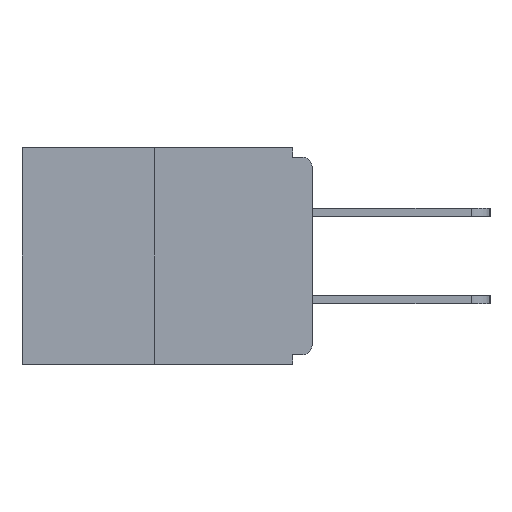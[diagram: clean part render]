
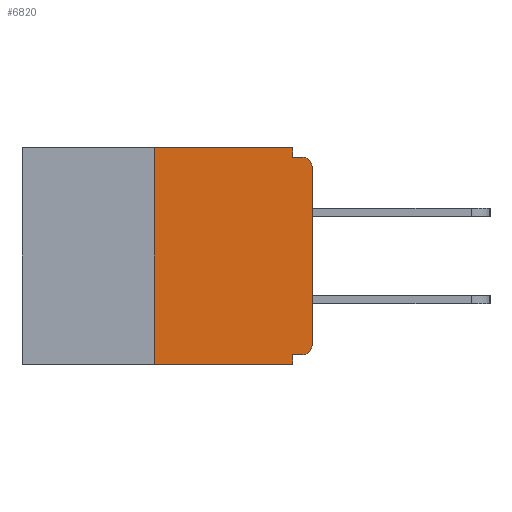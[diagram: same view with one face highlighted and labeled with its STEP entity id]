
A CAD part, left-side view. The second image highlights one B-rep face of the part: STEP entity #6820.
In plain terms, the highlighted planar face has unit normal (-1, 0, 0).
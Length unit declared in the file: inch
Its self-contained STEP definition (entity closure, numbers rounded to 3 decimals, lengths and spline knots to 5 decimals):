
#586 = VERTEX_POINT ( 'NONE', #4820 ) ;
#760 = CARTESIAN_POINT ( 'NONE',  ( 0., 0.015, -0.313 ) ) ;
#1252 = LINE ( 'NONE', #9778, #4649 ) ;
#1387 = VECTOR ( 'NONE', #11761, 39.37008 ) ;
#1599 = EDGE_CURVE ( 'NONE', #7360, #13210, #11874, .T. ) ;
#1698 = CARTESIAN_POINT ( 'NONE',  ( 0., 0.46, 0. ) ) ;
#1788 = EDGE_CURVE ( 'NONE', #4727, #586, #2448, .T. ) ;
#2043 = ORIENTED_EDGE ( 'NONE', *, *, #12614, .F. ) ;
#2048 = LINE ( 'NONE', #6075, #18670 ) ;
#2087 = VERTEX_POINT ( 'NONE', #13366 ) ;
#2448 = CIRCLE ( 'NONE', #17459, 0.015 ) ;
#2493 = DIRECTION ( 'NONE',  ( 0., 0., -1. ) ) ;
#2789 = DIRECTION ( 'NONE',  ( 0., -1., 0. ) ) ;
#2882 = DIRECTION ( 'NONE',  ( 0., 1., 0. ) ) ;
#3087 = VERTEX_POINT ( 'NONE', #14755 ) ;
#3408 = VERTEX_POINT ( 'NONE', #15895 ) ;
#3495 = LINE ( 'NONE', #4581, #8806 ) ;
#3751 = DIRECTION ( 'NONE',  ( -1., 0., 0. ) ) ;
#3957 = CIRCLE ( 'NONE', #9616, 0.015 ) ;
#4191 = CARTESIAN_POINT ( 'NONE',  ( 0., 0., -0.015 ) ) ;
#4308 = FACE_OUTER_BOUND ( 'NONE', #7816, .T. ) ;
#4376 = EDGE_CURVE ( 'NONE', #586, #6643, #3495, .T. ) ;
#4581 = CARTESIAN_POINT ( 'NONE',  ( 0., 0., 0. ) ) ;
#4649 = VECTOR ( 'NONE', #2882, 39.37008 ) ;
#4727 = VERTEX_POINT ( 'NONE', #10155 ) ;
#4807 = VECTOR ( 'NONE', #6513, 39.37008 ) ;
#4820 = CARTESIAN_POINT ( 'NONE',  ( 0., 0., -0.313 ) ) ;
#4939 = EDGE_CURVE ( 'NONE', #2087, #3087, #7409, .T. ) ;
#5169 = AXIS2_PLACEMENT_3D ( 'NONE', #1698, #14975, #18326 ) ;
#5762 = EDGE_CURVE ( 'NONE', #16862, #3087, #15166, .T. ) ;
#6075 = CARTESIAN_POINT ( 'NONE',  ( 0., 0.25, 0. ) ) ;
#6101 = ORIENTED_EDGE ( 'NONE', *, *, #18833, .F. ) ;
#6513 = DIRECTION ( 'NONE',  ( 0., 0., -1. ) ) ;
#6643 = VERTEX_POINT ( 'NONE', #14535 ) ;
#6654 = DIRECTION ( 'NONE',  ( 0., -1., 0. ) ) ;
#6820 = ADVANCED_FACE ( 'NONE', ( #4308 ), #10317, .F. ) ;
#6877 = CARTESIAN_POINT ( 'NONE',  ( 0., 0.031, 0. ) ) ;
#7171 = VECTOR ( 'NONE', #19897, 39.37008 ) ;
#7360 = VERTEX_POINT ( 'NONE', #11070 ) ;
#7409 = LINE ( 'NONE', #15191, #4807 ) ;
#7816 = EDGE_LOOP ( 'NONE', ( #19907, #16361, #17709, #11625, #6101, #13252, #16833, #12849, #2043, #17702 ) ) ;
#8806 = VECTOR ( 'NONE', #11123, 39.37008 ) ;
#9606 = CARTESIAN_POINT ( 'NONE',  ( 0., 0.015, -0.03 ) ) ;
#9616 = AXIS2_PLACEMENT_3D ( 'NONE', #9606, #19624, #2493 ) ;
#9634 = EDGE_CURVE ( 'NONE', #6643, #19759, #3957, .T. ) ;
#9778 = CARTESIAN_POINT ( 'NONE',  ( 0., 0., -0.328 ) ) ;
#9985 = CARTESIAN_POINT ( 'NONE',  ( 0., 0.46, 0. ) ) ;
#10155 = CARTESIAN_POINT ( 'NONE',  ( 0., 0.015, -0.328 ) ) ;
#10317 = PLANE ( 'NONE',  #5169 ) ;
#11070 = CARTESIAN_POINT ( 'NONE',  ( 0., 0.25, 0. ) ) ;
#11123 = DIRECTION ( 'NONE',  ( 0., 0., 1. ) ) ;
#11311 = VECTOR ( 'NONE', #6654, 39.37008 ) ;
#11625 = ORIENTED_EDGE ( 'NONE', *, *, #4939, .F. ) ;
#11761 = DIRECTION ( 'NONE',  ( 0., -1., 0. ) ) ;
#11773 = EDGE_CURVE ( 'NONE', #16862, #7360, #2048, .T. ) ;
#11859 = VECTOR ( 'NONE', #2789, 39.37008 ) ;
#11874 = LINE ( 'NONE', #9985, #11311 ) ;
#12005 = CARTESIAN_POINT ( 'NONE',  ( 0., 0.015, -0.015 ) ) ;
#12614 = EDGE_CURVE ( 'NONE', #3408, #19759, #20915, .T. ) ;
#12849 = ORIENTED_EDGE ( 'NONE', *, *, #9634, .T. ) ;
#13210 = VERTEX_POINT ( 'NONE', #6877 ) ;
#13252 = ORIENTED_EDGE ( 'NONE', *, *, #1788, .T. ) ;
#13366 = CARTESIAN_POINT ( 'NONE',  ( 0., 0.031, -0.328 ) ) ;
#13399 = LINE ( 'NONE', #18312, #7171 ) ;
#13590 = CARTESIAN_POINT ( 'NONE',  ( 0., 0.46, -0.343 ) ) ;
#14199 = DIRECTION ( 'NONE',  ( 0., 0., 1. ) ) ;
#14535 = CARTESIAN_POINT ( 'NONE',  ( 0., 0., -0.03 ) ) ;
#14755 = CARTESIAN_POINT ( 'NONE',  ( 0., 0.031, -0.343 ) ) ;
#14975 = DIRECTION ( 'NONE',  ( 1., 0., 0. ) ) ;
#15166 = LINE ( 'NONE', #13590, #1387 ) ;
#15191 = CARTESIAN_POINT ( 'NONE',  ( 0., 0.031, -0.343 ) ) ;
#15359 = DIRECTION ( 'NONE',  ( 0., 0., -1. ) ) ;
#15895 = CARTESIAN_POINT ( 'NONE',  ( 0., 0.031, -0.015 ) ) ;
#16361 = ORIENTED_EDGE ( 'NONE', *, *, #11773, .F. ) ;
#16833 = ORIENTED_EDGE ( 'NONE', *, *, #4376, .T. ) ;
#16862 = VERTEX_POINT ( 'NONE', #17544 ) ;
#17459 = AXIS2_PLACEMENT_3D ( 'NONE', #760, #3751, #15359 ) ;
#17544 = CARTESIAN_POINT ( 'NONE',  ( 0., 0.25, -0.343 ) ) ;
#17702 = ORIENTED_EDGE ( 'NONE', *, *, #20694, .F. ) ;
#17709 = ORIENTED_EDGE ( 'NONE', *, *, #5762, .T. ) ;
#18312 = CARTESIAN_POINT ( 'NONE',  ( 0., 0.031, 0. ) ) ;
#18326 = DIRECTION ( 'NONE',  ( 0., 0., -1. ) ) ;
#18670 = VECTOR ( 'NONE', #14199, 39.37008 ) ;
#18833 = EDGE_CURVE ( 'NONE', #4727, #2087, #1252, .T. ) ;
#19624 = DIRECTION ( 'NONE',  ( -1., 0., 0. ) ) ;
#19759 = VERTEX_POINT ( 'NONE', #12005 ) ;
#19897 = DIRECTION ( 'NONE',  ( 0., 0., -1. ) ) ;
#19907 = ORIENTED_EDGE ( 'NONE', *, *, #1599, .F. ) ;
#20694 = EDGE_CURVE ( 'NONE', #13210, #3408, #13399, .T. ) ;
#20915 = LINE ( 'NONE', #4191, #11859 ) ;
